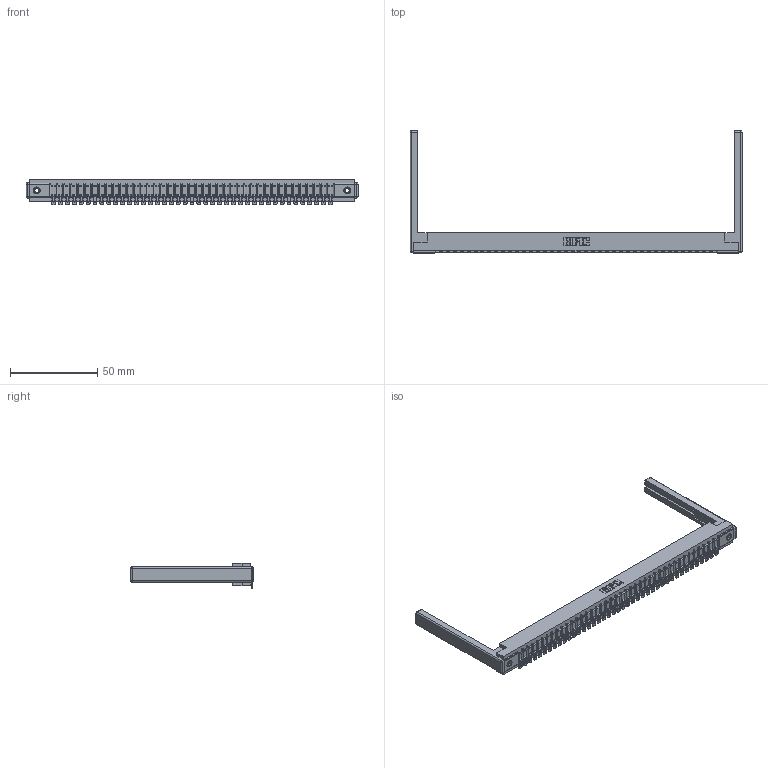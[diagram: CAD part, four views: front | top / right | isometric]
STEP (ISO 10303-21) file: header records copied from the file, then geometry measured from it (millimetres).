
FILE_DESCRIPTION (( 'STEP AP203' ), '1' );
FILE_NAME ('357-041-454-168.STEP', '2020-10-03T08:57:52', ( '' ), ( '' ), 'SwSTEP 2.0', 'SolidWorks 2020', '' );
FILE_SCHEMA (( 'CONFIG_CONTROL_DESIGN' ));
Length unit declared in the file: inch
Products named in the file (5): 357-041-454-168; 345-250-001_345-250-001-102; 307-290-002_554; 307-220-068; 307 Part_.156 Dia Mounting Holes
Assembly tree (46 placements, depth 2):
  357-041-454-168
    307 Part_.156 Dia Mounting Holes
    307-290-002_554  x41
    307-220-068  x2
    345-250-001_345-250-001-102  x2
Bounding box: 189.89 x 69.98 x 14.52 mm (x, y, z)
Volume: 24705.6 mm3; surface area: 29656.6 mm2
Topology: 46 solids, 46 shells, 3635 faces, 11086 edges, 7256 vertices
Faces by surface type: plane 2044, cylinder 1483, sphere 92, cone 12, torus 4
Entity records: 38996 total; most frequent: CARTESIAN_POINT 6543, ORIENTED_EDGE 6522, DIRECTION 6381, EDGE_CURVE 3261, VECTOR 2489, LINE 2489, VERTEX_POINT 2108, AXIS2_PLACEMENT_3D 1946
